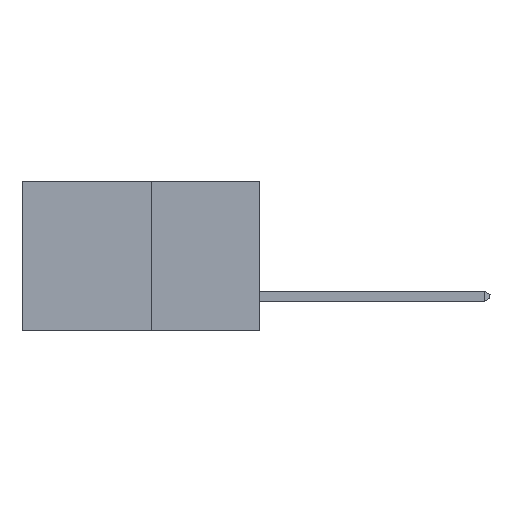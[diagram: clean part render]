
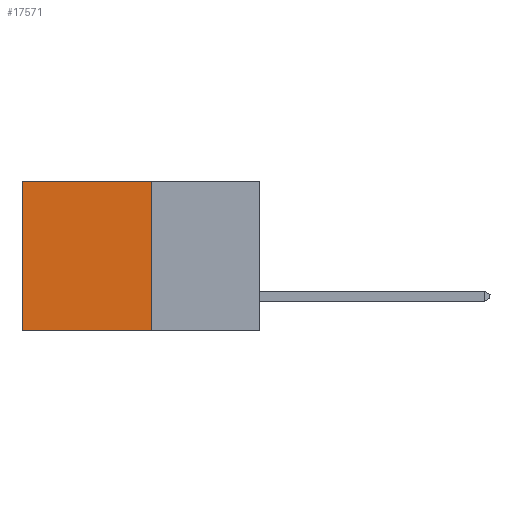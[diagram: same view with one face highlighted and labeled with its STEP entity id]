
A CAD part, left-side view. The second image highlights one B-rep face of the part: STEP entity #17571.
In plain terms, the highlighted planar face has unit normal (-1, 0, 0).
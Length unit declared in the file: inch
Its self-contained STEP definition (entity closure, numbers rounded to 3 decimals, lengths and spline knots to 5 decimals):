
#85 = DIRECTION ( 'NONE',  ( 0., 0., -1. ) ) ;
#270 = AXIS2_PLACEMENT_3D ( 'NONE', #5594, #21559, #11150 ) ;
#1072 = CARTESIAN_POINT ( 'NONE',  ( 0.277, 0.59, -0.37 ) ) ;
#2301 = ORIENTED_EDGE ( 'NONE', *, *, #11169, .T. ) ;
#2318 = LINE ( 'NONE', #4499, #11525 ) ;
#3170 = CARTESIAN_POINT ( 'NONE',  ( 0.277, 0.27, 0. ) ) ;
#3263 = LINE ( 'NONE', #12935, #8743 ) ;
#4499 = CARTESIAN_POINT ( 'NONE',  ( 0.277, 0.27, 0. ) ) ;
#5487 = EDGE_LOOP ( 'NONE', ( #2301, #13878, #21252, #15720 ) ) ;
#5594 = CARTESIAN_POINT ( 'NONE',  ( 0.277, 0.27, -0.37 ) ) ;
#6234 = VERTEX_POINT ( 'NONE', #1072 ) ;
#7086 = VECTOR ( 'NONE', #8414, 39.37008 ) ;
#7252 = EDGE_CURVE ( 'NONE', #21801, #6234, #16566, .T. ) ;
#8414 = DIRECTION ( 'NONE',  ( 0., 1., 0. ) ) ;
#8743 = VECTOR ( 'NONE', #85, 39.37008 ) ;
#9288 = PLANE ( 'NONE',  #270 ) ;
#9687 = CARTESIAN_POINT ( 'NONE',  ( 0.277, 0.27, -0.37 ) ) ;
#9745 = CARTESIAN_POINT ( 'NONE',  ( 0.277, 0.59, 0. ) ) ;
#11150 = DIRECTION ( 'NONE',  ( 0., 0., -1. ) ) ;
#11169 = EDGE_CURVE ( 'NONE', #16440, #6234, #14823, .T. ) ;
#11525 = VECTOR ( 'NONE', #18766, 39.37008 ) ;
#12087 = CARTESIAN_POINT ( 'NONE',  ( 0.277, 0.27, -0.37 ) ) ;
#12130 = EDGE_CURVE ( 'NONE', #12310, #16440, #2318, .T. ) ;
#12310 = VERTEX_POINT ( 'NONE', #3170 ) ;
#12935 = CARTESIAN_POINT ( 'NONE',  ( 0.277, 0.27, -0.37 ) ) ;
#12996 = FACE_OUTER_BOUND ( 'NONE', #5487, .T. ) ;
#13878 = ORIENTED_EDGE ( 'NONE', *, *, #7252, .F. ) ;
#14823 = LINE ( 'NONE', #19589, #18392 ) ;
#15720 = ORIENTED_EDGE ( 'NONE', *, *, #12130, .T. ) ;
#16440 = VERTEX_POINT ( 'NONE', #9745 ) ;
#16566 = LINE ( 'NONE', #9687, #7086 ) ;
#17571 = ADVANCED_FACE ( 'NONE', ( #12996 ), #9288, .F. ) ;
#17579 = EDGE_CURVE ( 'NONE', #12310, #21801, #3263, .T. ) ;
#18392 = VECTOR ( 'NONE', #21313, 39.37008 ) ;
#18766 = DIRECTION ( 'NONE',  ( 0., 1., 0. ) ) ;
#19589 = CARTESIAN_POINT ( 'NONE',  ( 0.277, 0.59, -0.37 ) ) ;
#21252 = ORIENTED_EDGE ( 'NONE', *, *, #17579, .F. ) ;
#21313 = DIRECTION ( 'NONE',  ( 0., 0., -1. ) ) ;
#21559 = DIRECTION ( 'NONE',  ( 1., 0., 0. ) ) ;
#21801 = VERTEX_POINT ( 'NONE', #12087 ) ;
